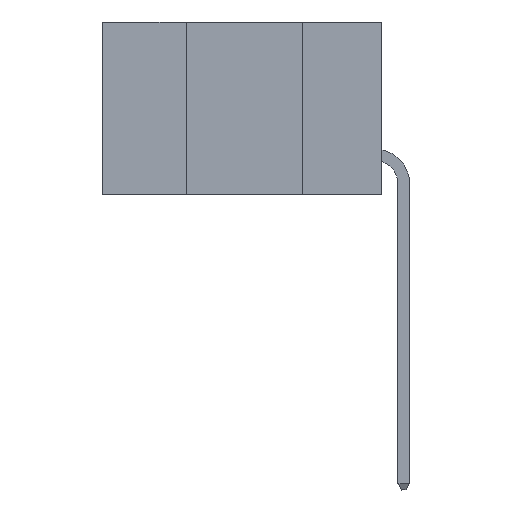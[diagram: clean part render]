
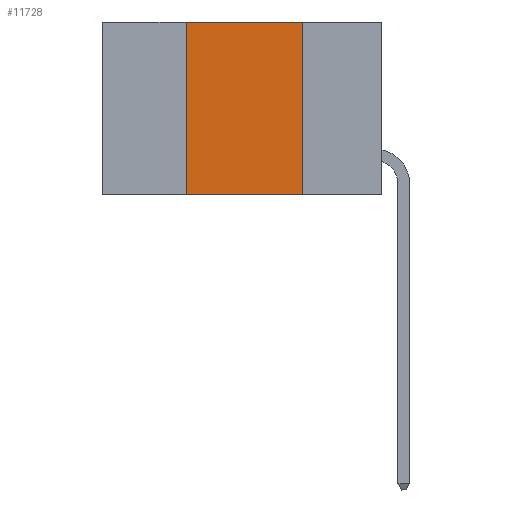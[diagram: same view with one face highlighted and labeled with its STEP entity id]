
A CAD part, left-side view. The second image highlights one B-rep face of the part: STEP entity #11728.
In plain terms, the highlighted planar face has unit normal (-1, 0, 0).
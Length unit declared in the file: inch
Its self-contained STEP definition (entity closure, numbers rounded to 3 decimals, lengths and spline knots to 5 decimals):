
#153 = VECTOR ( 'NONE', #3496, 39.37008 ) ;
#474 = LINE ( 'NONE', #17344, #17506 ) ;
#637 = CARTESIAN_POINT ( 'NONE',  ( 0., 0.6, 0. ) ) ;
#698 = VERTEX_POINT ( 'NONE', #4547 ) ;
#727 = DIRECTION ( 'NONE',  ( 0., 0., 1. ) ) ;
#2032 = EDGE_CURVE ( 'NONE', #16578, #698, #3264, .T. ) ;
#2958 = ORIENTED_EDGE ( 'NONE', *, *, #14068, .T. ) ;
#3264 = LINE ( 'NONE', #15628, #16496 ) ;
#3459 = ORIENTED_EDGE ( 'NONE', *, *, #7736, .F. ) ;
#3496 = DIRECTION ( 'NONE',  ( 0., -1., 0. ) ) ;
#3860 = VERTEX_POINT ( 'NONE', #16967 ) ;
#4151 = LINE ( 'NONE', #11930, #5634 ) ;
#4247 = ORIENTED_EDGE ( 'NONE', *, *, #7772, .F. ) ;
#4547 = CARTESIAN_POINT ( 'NONE',  ( 0., 0.42, 0. ) ) ;
#5634 = VECTOR ( 'NONE', #10643, 39.37008 ) ;
#6185 = DIRECTION ( 'NONE',  ( 0., -1., 0. ) ) ;
#6458 = AXIS2_PLACEMENT_3D ( 'NONE', #15706, #14417, #11656 ) ;
#7736 = EDGE_CURVE ( 'NONE', #698, #3860, #17615, .T. ) ;
#7772 = EDGE_CURVE ( 'NONE', #3860, #13677, #4151, .T. ) ;
#9560 = CARTESIAN_POINT ( 'NONE',  ( 0., 0.42, -0.37 ) ) ;
#9902 = PLANE ( 'NONE',  #6458 ) ;
#10643 = DIRECTION ( 'NONE',  ( 0., 0., -1. ) ) ;
#11168 = CARTESIAN_POINT ( 'NONE',  ( 0., 0.17, -0.37 ) ) ;
#11250 = ORIENTED_EDGE ( 'NONE', *, *, #2032, .F. ) ;
#11656 = DIRECTION ( 'NONE',  ( 0., 0., -1. ) ) ;
#11728 = ADVANCED_FACE ( 'NONE', ( #13569 ), #9902, .F. ) ;
#11930 = CARTESIAN_POINT ( 'NONE',  ( 0., 0.17, 0. ) ) ;
#13569 = FACE_OUTER_BOUND ( 'NONE', #16735, .T. ) ;
#13677 = VERTEX_POINT ( 'NONE', #11168 ) ;
#14068 = EDGE_CURVE ( 'NONE', #16578, #13677, #474, .T. ) ;
#14417 = DIRECTION ( 'NONE',  ( 1., 0., 0. ) ) ;
#15628 = CARTESIAN_POINT ( 'NONE',  ( 0., 0.42, 0. ) ) ;
#15706 = CARTESIAN_POINT ( 'NONE',  ( 0., 0.6, 0. ) ) ;
#16496 = VECTOR ( 'NONE', #727, 39.37008 ) ;
#16578 = VERTEX_POINT ( 'NONE', #9560 ) ;
#16735 = EDGE_LOOP ( 'NONE', ( #4247, #3459, #11250, #2958 ) ) ;
#16967 = CARTESIAN_POINT ( 'NONE',  ( 0., 0.17, 0. ) ) ;
#17344 = CARTESIAN_POINT ( 'NONE',  ( 0., 0.6, -0.37 ) ) ;
#17506 = VECTOR ( 'NONE', #6185, 39.37008 ) ;
#17615 = LINE ( 'NONE', #637, #153 ) ;
